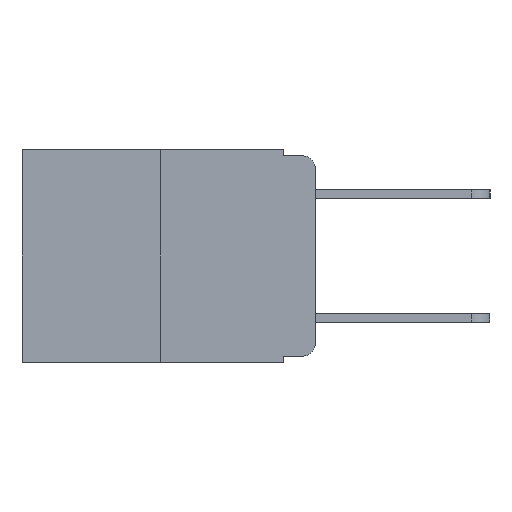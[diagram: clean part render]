
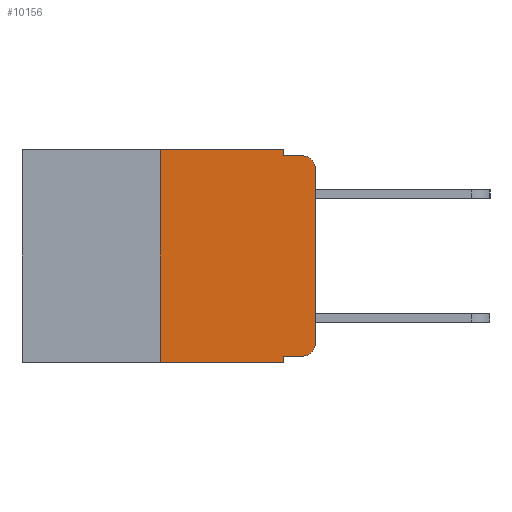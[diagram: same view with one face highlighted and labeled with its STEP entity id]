
A CAD part, left-side view. The second image highlights one B-rep face of the part: STEP entity #10156.
In plain terms, the highlighted planar face has unit normal (-1, 0, 0).
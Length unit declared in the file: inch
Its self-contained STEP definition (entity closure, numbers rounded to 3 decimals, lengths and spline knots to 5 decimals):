
#215 = LINE ( 'NONE', #4089, #13402 ) ;
#231 = ORIENTED_EDGE ( 'NONE', *, *, #17255, .F. ) ;
#292 = LINE ( 'NONE', #18466, #8840 ) ;
#362 = CARTESIAN_POINT ( 'NONE',  ( 0., 0.051, -0.333 ) ) ;
#759 = DIRECTION ( 'NONE',  ( 0., 0., -1. ) ) ;
#1370 = DIRECTION ( 'NONE',  ( 1., 0., 0. ) ) ;
#1686 = ORIENTED_EDGE ( 'NONE', *, *, #11300, .T. ) ;
#1938 = VERTEX_POINT ( 'NONE', #10425 ) ;
#1952 = ORIENTED_EDGE ( 'NONE', *, *, #6826, .T. ) ;
#2144 = DIRECTION ( 'NONE',  ( 0., -1., 0. ) ) ;
#2199 = CARTESIAN_POINT ( 'NONE',  ( 0., 0.051, 0. ) ) ;
#2539 = CARTESIAN_POINT ( 'NONE',  ( 0., 0.25, -0.343 ) ) ;
#3277 = LINE ( 'NONE', #15527, #19449 ) ;
#3284 = CARTESIAN_POINT ( 'NONE',  ( 0., 0.02, -0.333 ) ) ;
#3388 = DIRECTION ( 'NONE',  ( -1., 0., 0. ) ) ;
#3502 = CARTESIAN_POINT ( 'NONE',  ( 0., 0.02, -0.01 ) ) ;
#3545 = VERTEX_POINT ( 'NONE', #3502 ) ;
#4068 = AXIS2_PLACEMENT_3D ( 'NONE', #19724, #10857, #759 ) ;
#4089 = CARTESIAN_POINT ( 'NONE',  ( 0., 0.051, 0. ) ) ;
#4220 = EDGE_CURVE ( 'NONE', #1938, #3545, #16556, .T. ) ;
#4347 = ORIENTED_EDGE ( 'NONE', *, *, #20338, .F. ) ;
#4440 = VECTOR ( 'NONE', #6980, 39.37008 ) ;
#4975 = VERTEX_POINT ( 'NONE', #20248 ) ;
#5336 = CARTESIAN_POINT ( 'NONE',  ( 0., 0., -0.03 ) ) ;
#5379 = EDGE_CURVE ( 'NONE', #16366, #3545, #8096, .T. ) ;
#5574 = ORIENTED_EDGE ( 'NONE', *, *, #6539, .T. ) ;
#5917 = LINE ( 'NONE', #362, #10317 ) ;
#6339 = CARTESIAN_POINT ( 'NONE',  ( 0., 0.051, 0. ) ) ;
#6367 = VERTEX_POINT ( 'NONE', #3284 ) ;
#6449 = AXIS2_PLACEMENT_3D ( 'NONE', #13175, #3388, #14676 ) ;
#6539 = EDGE_CURVE ( 'NONE', #19936, #16366, #16710, .T. ) ;
#6826 = EDGE_CURVE ( 'NONE', #12639, #8111, #3277, .T. ) ;
#6980 = DIRECTION ( 'NONE',  ( 0., -1., 0. ) ) ;
#6985 = CARTESIAN_POINT ( 'NONE',  ( 0., 0.051, -0.01 ) ) ;
#7367 = ORIENTED_EDGE ( 'NONE', *, *, #13337, .F. ) ;
#7821 = DIRECTION ( 'NONE',  ( 0., -1., 0. ) ) ;
#8096 = CIRCLE ( 'NONE', #4068, 0.02 ) ;
#8111 = VERTEX_POINT ( 'NONE', #19666 ) ;
#8840 = VECTOR ( 'NONE', #15529, 39.37008 ) ;
#9708 = VECTOR ( 'NONE', #12278, 39.37008 ) ;
#9859 = FACE_OUTER_BOUND ( 'NONE', #15466, .T. ) ;
#10156 = ADVANCED_FACE ( 'NONE', ( #9859 ), #20231, .F. ) ;
#10253 = EDGE_CURVE ( 'NONE', #6367, #19936, #16032, .T. ) ;
#10317 = VECTOR ( 'NONE', #2144, 39.37008 ) ;
#10402 = DIRECTION ( 'NONE',  ( 0., 0., 1. ) ) ;
#10425 = CARTESIAN_POINT ( 'NONE',  ( 0., 0.051, -0.01 ) ) ;
#10687 = CARTESIAN_POINT ( 'NONE',  ( 0., 0.473, 0. ) ) ;
#10857 = DIRECTION ( 'NONE',  ( -1., 0., 0. ) ) ;
#11300 = EDGE_CURVE ( 'NONE', #16207, #6367, #5917, .T. ) ;
#11318 = CARTESIAN_POINT ( 'NONE',  ( 0., 0.473, 0. ) ) ;
#12278 = DIRECTION ( 'NONE',  ( 0., -1., 0. ) ) ;
#12639 = VERTEX_POINT ( 'NONE', #2539 ) ;
#12776 = VECTOR ( 'NONE', #10402, 39.37008 ) ;
#12914 = DIRECTION ( 'NONE',  ( 0., 0., -1. ) ) ;
#13136 = ORIENTED_EDGE ( 'NONE', *, *, #5379, .T. ) ;
#13175 = CARTESIAN_POINT ( 'NONE',  ( 0., 0.02, -0.313 ) ) ;
#13337 = EDGE_CURVE ( 'NONE', #16207, #8111, #14999, .T. ) ;
#13402 = VECTOR ( 'NONE', #16737, 39.37008 ) ;
#13410 = CARTESIAN_POINT ( 'NONE',  ( 0., 0., 0. ) ) ;
#13424 = ORIENTED_EDGE ( 'NONE', *, *, #10253, .T. ) ;
#13803 = LINE ( 'NONE', #10687, #9708 ) ;
#14676 = DIRECTION ( 'NONE',  ( 0., 0., -1. ) ) ;
#14969 = ORIENTED_EDGE ( 'NONE', *, *, #19245, .F. ) ;
#14999 = LINE ( 'NONE', #6339, #18410 ) ;
#15097 = VERTEX_POINT ( 'NONE', #2199 ) ;
#15466 = EDGE_LOOP ( 'NONE', ( #5574, #13136, #19206, #14969, #4347, #231, #1952, #7367, #1686, #13424 ) ) ;
#15527 = CARTESIAN_POINT ( 'NONE',  ( 0., 0.473, -0.343 ) ) ;
#15529 = DIRECTION ( 'NONE',  ( 0., 0., 1. ) ) ;
#16032 = CIRCLE ( 'NONE', #6449, 0.02 ) ;
#16207 = VERTEX_POINT ( 'NONE', #17412 ) ;
#16366 = VERTEX_POINT ( 'NONE', #5336 ) ;
#16556 = LINE ( 'NONE', #6985, #4440 ) ;
#16710 = LINE ( 'NONE', #13410, #12776 ) ;
#16737 = DIRECTION ( 'NONE',  ( 0., 0., -1. ) ) ;
#17185 = AXIS2_PLACEMENT_3D ( 'NONE', #11318, #1370, #12914 ) ;
#17255 = EDGE_CURVE ( 'NONE', #12639, #4975, #292, .T. ) ;
#17412 = CARTESIAN_POINT ( 'NONE',  ( 0., 0.051, -0.333 ) ) ;
#18410 = VECTOR ( 'NONE', #20045, 39.37008 ) ;
#18466 = CARTESIAN_POINT ( 'NONE',  ( 0., 0.25, 0. ) ) ;
#18631 = CARTESIAN_POINT ( 'NONE',  ( 0., 0., -0.313 ) ) ;
#19206 = ORIENTED_EDGE ( 'NONE', *, *, #4220, .F. ) ;
#19245 = EDGE_CURVE ( 'NONE', #15097, #1938, #215, .T. ) ;
#19449 = VECTOR ( 'NONE', #7821, 39.37008 ) ;
#19666 = CARTESIAN_POINT ( 'NONE',  ( 0., 0.051, -0.343 ) ) ;
#19724 = CARTESIAN_POINT ( 'NONE',  ( 0., 0.02, -0.03 ) ) ;
#19936 = VERTEX_POINT ( 'NONE', #18631 ) ;
#20045 = DIRECTION ( 'NONE',  ( 0., 0., -1. ) ) ;
#20231 = PLANE ( 'NONE',  #17185 ) ;
#20248 = CARTESIAN_POINT ( 'NONE',  ( 0., 0.25, 0. ) ) ;
#20338 = EDGE_CURVE ( 'NONE', #4975, #15097, #13803, .T. ) ;
